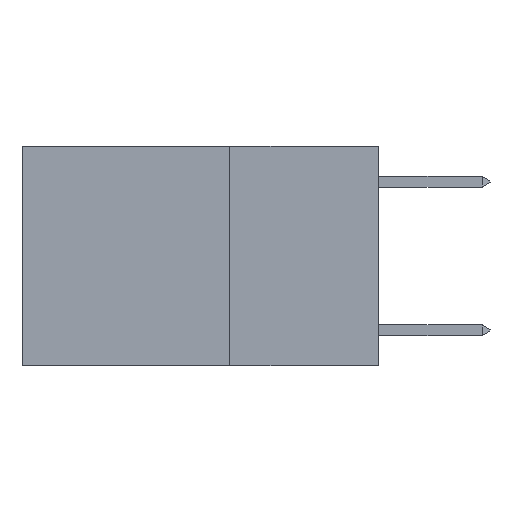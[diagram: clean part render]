
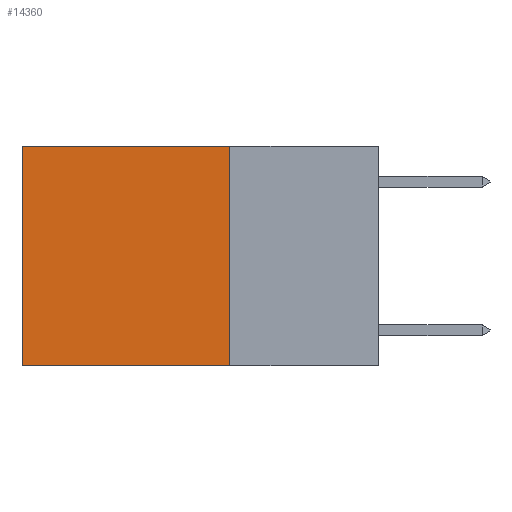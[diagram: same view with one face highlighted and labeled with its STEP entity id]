
A CAD part, left-side view. The second image highlights one B-rep face of the part: STEP entity #14360.
In plain terms, the highlighted planar face has unit normal (-1, 0, 0).
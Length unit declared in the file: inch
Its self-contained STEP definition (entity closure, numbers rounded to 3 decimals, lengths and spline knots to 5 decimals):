
#550 = CARTESIAN_POINT ( 'NONE',  ( 0.2625, 0.25, -0.37 ) ) ;
#961 = VERTEX_POINT ( 'NONE', #5178 ) ;
#1941 = EDGE_LOOP ( 'NONE', ( #15632, #19755, #4952, #23583 ) ) ;
#2479 = DIRECTION ( 'NONE',  ( 0., 1., 0. ) ) ;
#4069 = DIRECTION ( 'NONE',  ( 0., 0., -1. ) ) ;
#4090 = VECTOR ( 'NONE', #2479, 39.37008 ) ;
#4315 = DIRECTION ( 'NONE',  ( 1., 0., 0. ) ) ;
#4952 = ORIENTED_EDGE ( 'NONE', *, *, #11437, .F. ) ;
#5169 = CARTESIAN_POINT ( 'NONE',  ( 0.2625, 0.25, -0.37 ) ) ;
#5178 = CARTESIAN_POINT ( 'NONE',  ( 0.2625, 0.6, 0. ) ) ;
#5307 = CARTESIAN_POINT ( 'NONE',  ( 0.2625, 0.25, 0. ) ) ;
#6000 = VECTOR ( 'NONE', #4069, 39.37008 ) ;
#6235 = CARTESIAN_POINT ( 'NONE',  ( 0.2625, 0.25, 0. ) ) ;
#6353 = CARTESIAN_POINT ( 'NONE',  ( 0.2625, 0.25, 0. ) ) ;
#11280 = VERTEX_POINT ( 'NONE', #19382 ) ;
#11437 = EDGE_CURVE ( 'NONE', #19445, #17278, #23629, .T. ) ;
#11621 = DIRECTION ( 'NONE',  ( 0., 0., -1. ) ) ;
#12358 = VECTOR ( 'NONE', #19858, 39.37008 ) ;
#12967 = EDGE_CURVE ( 'NONE', #17278, #11280, #20809, .T. ) ;
#13344 = PLANE ( 'NONE',  #21673 ) ;
#13427 = LINE ( 'NONE', #20438, #4090 ) ;
#14360 = ADVANCED_FACE ( 'NONE', ( #20695 ), #13344, .F. ) ;
#15632 = ORIENTED_EDGE ( 'NONE', *, *, #20866, .T. ) ;
#17278 = VERTEX_POINT ( 'NONE', #5169 ) ;
#19113 = DIRECTION ( 'NONE',  ( 0., 1., 0. ) ) ;
#19382 = CARTESIAN_POINT ( 'NONE',  ( 0.2625, 0.6, -0.37 ) ) ;
#19445 = VERTEX_POINT ( 'NONE', #6235 ) ;
#19733 = VECTOR ( 'NONE', #19113, 39.37008 ) ;
#19755 = ORIENTED_EDGE ( 'NONE', *, *, #12967, .F. ) ;
#19858 = DIRECTION ( 'NONE',  ( 0., 0., -1. ) ) ;
#20438 = CARTESIAN_POINT ( 'NONE',  ( 0.2625, 0.25, 0. ) ) ;
#20695 = FACE_OUTER_BOUND ( 'NONE', #1941, .T. ) ;
#20809 = LINE ( 'NONE', #550, #19733 ) ;
#20866 = EDGE_CURVE ( 'NONE', #961, #11280, #22519, .T. ) ;
#21406 = EDGE_CURVE ( 'NONE', #19445, #961, #13427, .T. ) ;
#21673 = AXIS2_PLACEMENT_3D ( 'NONE', #6353, #4315, #11621 ) ;
#22519 = LINE ( 'NONE', #22882, #6000 ) ;
#22882 = CARTESIAN_POINT ( 'NONE',  ( 0.2625, 0.6, 0. ) ) ;
#23583 = ORIENTED_EDGE ( 'NONE', *, *, #21406, .T. ) ;
#23629 = LINE ( 'NONE', #5307, #12358 ) ;
